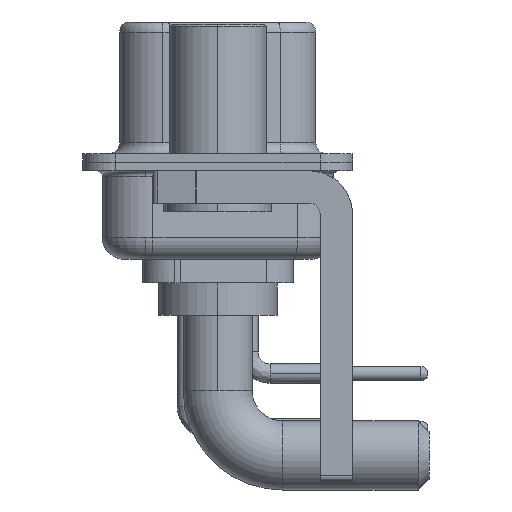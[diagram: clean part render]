
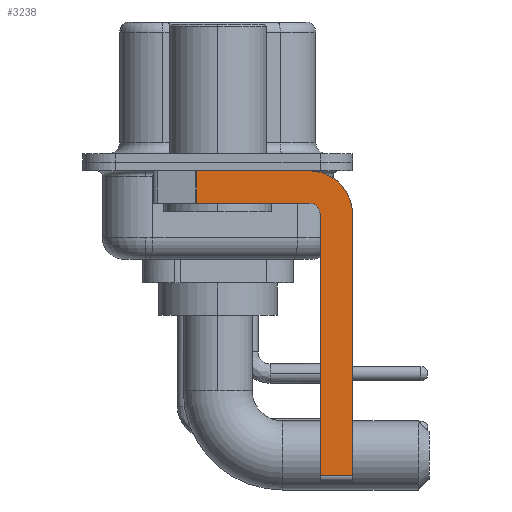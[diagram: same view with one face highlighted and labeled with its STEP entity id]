
A CAD part, left-side view. The second image highlights one B-rep face of the part: STEP entity #3238.
In plain terms, the highlighted planar face has unit normal (-1, 0, 0).
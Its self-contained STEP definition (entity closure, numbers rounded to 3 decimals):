
#189 = DIRECTION ( 'NONE',  ( 0., 0., -1. ) ) ;
#902 = CARTESIAN_POINT ( 'NONE',  ( -2.9, 3., -0.4 ) ) ;
#1049 = EDGE_LOOP ( 'NONE', ( #24657, #13267, #15082, #23251, #21633, #12545, #6759, #4295 ) ) ;
#2157 = CARTESIAN_POINT ( 'NONE',  ( -2.9, -6.25, -14.55 ) ) ;
#2295 = DIRECTION ( 'NONE',  ( 0., -1., 0. ) ) ;
#2638 = DIRECTION ( 'NONE',  ( 0., 0., -1. ) ) ;
#2953 = VERTEX_POINT ( 'NONE', #2157 ) ;
#3238 = ADVANCED_FACE ( 'NONE', ( #11082 ), #15376, .F. ) ;
#3288 = CARTESIAN_POINT ( 'NONE',  ( -2.9, -4.25, -14.55 ) ) ;
#3562 = VECTOR ( 'NONE', #22446, 1000. ) ;
#4295 = ORIENTED_EDGE ( 'NONE', *, *, #20221, .F. ) ;
#4740 = CARTESIAN_POINT ( 'NONE',  ( -2.9, -4.75, -14.8 ) ) ;
#4802 = AXIS2_PLACEMENT_3D ( 'NONE', #18779, #17140, #11461 ) ;
#5234 = CARTESIAN_POINT ( 'NONE',  ( -2.9, -4.75, -14.55 ) ) ;
#5731 = CIRCLE ( 'NONE', #22687, 2. ) ;
#5779 = VERTEX_POINT ( 'NONE', #24458 ) ;
#5885 = VECTOR ( 'NONE', #2295, 1000. ) ;
#6008 = VECTOR ( 'NONE', #19554, 1000. ) ;
#6759 = ORIENTED_EDGE ( 'NONE', *, *, #21313, .F. ) ;
#7191 = CARTESIAN_POINT ( 'NONE',  ( -2.9, -6.25, -2.4 ) ) ;
#7895 = EDGE_CURVE ( 'NONE', #19109, #5779, #22059, .T. ) ;
#8010 = LINE ( 'NONE', #9899, #12896 ) ;
#8544 = LINE ( 'NONE', #4740, #6008 ) ;
#9371 = CARTESIAN_POINT ( 'NONE',  ( -2.9, -4.25, -1.9 ) ) ;
#9445 = CARTESIAN_POINT ( 'NONE',  ( -2.9, 0.978, -0.4 ) ) ;
#9870 = VERTEX_POINT ( 'NONE', #19205 ) ;
#9899 = CARTESIAN_POINT ( 'NONE',  ( -2.9, 0.978, -1.9 ) ) ;
#10166 = VERTEX_POINT ( 'NONE', #9445 ) ;
#11082 = FACE_OUTER_BOUND ( 'NONE', #1049, .T. ) ;
#11461 = DIRECTION ( 'NONE',  ( 0., 0., -1. ) ) ;
#11988 = EDGE_CURVE ( 'NONE', #10166, #19714, #19596, .T. ) ;
#12145 = CARTESIAN_POINT ( 'NONE',  ( -2.9, -4.25, -0.4 ) ) ;
#12545 = ORIENTED_EDGE ( 'NONE', *, *, #19948, .T. ) ;
#12555 = CIRCLE ( 'NONE', #16193, 0.5 ) ;
#12891 = DIRECTION ( 'NONE',  ( 0., 0., -1. ) ) ;
#12896 = VECTOR ( 'NONE', #189, 1000. ) ;
#13267 = ORIENTED_EDGE ( 'NONE', *, *, #17461, .T. ) ;
#14093 = VECTOR ( 'NONE', #12891, 1000. ) ;
#14136 = CARTESIAN_POINT ( 'NONE',  ( -2.9, -4.25, -2.4 ) ) ;
#14356 = VERTEX_POINT ( 'NONE', #5234 ) ;
#15082 = ORIENTED_EDGE ( 'NONE', *, *, #7895, .F. ) ;
#15376 = PLANE ( 'NONE',  #4802 ) ;
#16193 = AXIS2_PLACEMENT_3D ( 'NONE', #23915, #16592, #18596 ) ;
#16522 = CARTESIAN_POINT ( 'NONE',  ( -2.9, -4.25, -1.9 ) ) ;
#16592 = DIRECTION ( 'NONE',  ( -1., 0., 0. ) ) ;
#16930 = LINE ( 'NONE', #3288, #19047 ) ;
#17140 = DIRECTION ( 'NONE',  ( 1., 0., 0. ) ) ;
#17211 = CARTESIAN_POINT ( 'NONE',  ( -2.9, -6.25, -2.4 ) ) ;
#17461 = EDGE_CURVE ( 'NONE', #10166, #5779, #8010, .T. ) ;
#18596 = DIRECTION ( 'NONE',  ( 0., 0., 1. ) ) ;
#18697 = DIRECTION ( 'NONE',  ( 0., -1., 0. ) ) ;
#18779 = CARTESIAN_POINT ( 'NONE',  ( -2.9, -4.25, -2.4 ) ) ;
#19047 = VECTOR ( 'NONE', #18697, 1000. ) ;
#19109 = VERTEX_POINT ( 'NONE', #9371 ) ;
#19205 = CARTESIAN_POINT ( 'NONE',  ( -2.9, -4.75, -2.4 ) ) ;
#19554 = DIRECTION ( 'NONE',  ( 0., 0., 1. ) ) ;
#19596 = LINE ( 'NONE', #902, #5885 ) ;
#19714 = VERTEX_POINT ( 'NONE', #12145 ) ;
#19948 = EDGE_CURVE ( 'NONE', #14356, #2953, #16930, .T. ) ;
#20221 = EDGE_CURVE ( 'NONE', #19714, #22830, #5731, .T. ) ;
#20800 = EDGE_CURVE ( 'NONE', #14356, #9870, #8544, .T. ) ;
#21313 = EDGE_CURVE ( 'NONE', #22830, #2953, #24753, .T. ) ;
#21633 = ORIENTED_EDGE ( 'NONE', *, *, #20800, .F. ) ;
#22059 = LINE ( 'NONE', #16522, #3562 ) ;
#22446 = DIRECTION ( 'NONE',  ( 0., 1., 0. ) ) ;
#22687 = AXIS2_PLACEMENT_3D ( 'NONE', #14136, #23983, #2638 ) ;
#22830 = VERTEX_POINT ( 'NONE', #17211 ) ;
#23251 = ORIENTED_EDGE ( 'NONE', *, *, #23324, .F. ) ;
#23324 = EDGE_CURVE ( 'NONE', #9870, #19109, #12555, .T. ) ;
#23915 = CARTESIAN_POINT ( 'NONE',  ( -2.9, -4.25, -2.4 ) ) ;
#23983 = DIRECTION ( 'NONE',  ( 1., 0., 0. ) ) ;
#24458 = CARTESIAN_POINT ( 'NONE',  ( -2.9, 0.978, -1.9 ) ) ;
#24657 = ORIENTED_EDGE ( 'NONE', *, *, #11988, .F. ) ;
#24753 = LINE ( 'NONE', #7191, #14093 ) ;
